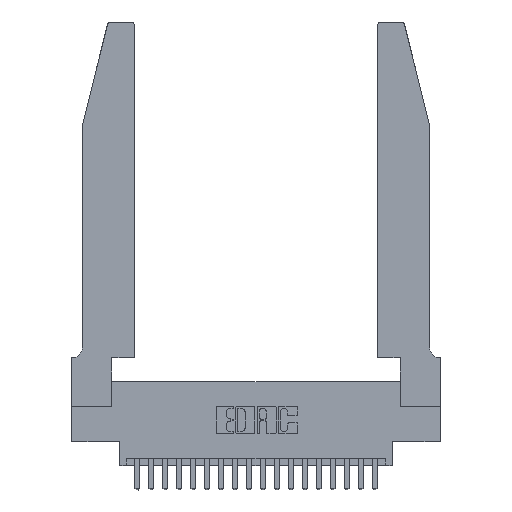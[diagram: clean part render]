
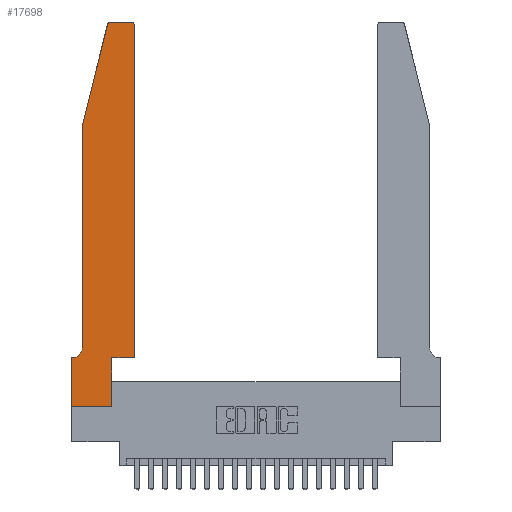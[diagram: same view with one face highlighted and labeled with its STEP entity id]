
A CAD part, top view. The second image highlights one B-rep face of the part: STEP entity #17698.
In plain terms, the highlighted planar face has unit normal (0, 0, 1).
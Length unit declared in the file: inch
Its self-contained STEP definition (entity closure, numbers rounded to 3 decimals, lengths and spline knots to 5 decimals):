
#39 = VERTEX_POINT ( 'NONE', #20597 ) ;
#129 = DIRECTION ( 'NONE',  ( 1., 0., 0. ) ) ;
#146 = LINE ( 'NONE', #2811, #18498 ) ;
#521 = EDGE_CURVE ( 'NONE', #4334, #8760, #20415, .T. ) ;
#886 = CARTESIAN_POINT ( 'NONE',  ( 0.4505, 0.35, 0.37 ) ) ;
#963 = FACE_OUTER_BOUND ( 'NONE', #15360, .T. ) ;
#997 = CARTESIAN_POINT ( 'NONE',  ( 0.0755, 2., 0.37 ) ) ;
#1043 = DIRECTION ( 'NONE',  ( -1., 0., 0. ) ) ;
#1057 = LINE ( 'NONE', #11172, #6440 ) ;
#1063 = DIRECTION ( 'NONE',  ( -1., 0., 0. ) ) ;
#1068 = VERTEX_POINT ( 'NONE', #13540 ) ;
#1978 = ORIENTED_EDGE ( 'NONE', *, *, #2964, .T. ) ;
#2248 = ORIENTED_EDGE ( 'NONE', *, *, #521, .T. ) ;
#2515 = LINE ( 'NONE', #7045, #15739 ) ;
#2811 = CARTESIAN_POINT ( 'NONE',  ( 0.0755, 0.35, 0.37 ) ) ;
#2919 = CIRCLE ( 'NONE', #5789, 0.07 ) ;
#2964 = EDGE_CURVE ( 'NONE', #6423, #7801, #2919, .T. ) ;
#3041 = DIRECTION ( 'NONE',  ( 0., 1., 0. ) ) ;
#3249 = ORIENTED_EDGE ( 'NONE', *, *, #6987, .T. ) ;
#3311 = LINE ( 'NONE', #997, #21157 ) ;
#4334 = VERTEX_POINT ( 'NONE', #6248 ) ;
#4437 = CARTESIAN_POINT ( 'NONE',  ( 0.4205, 2.75, 0.37 ) ) ;
#4625 = CARTESIAN_POINT ( 'NONE',  ( 0., 0.35, 0.37 ) ) ;
#4846 = VERTEX_POINT ( 'NONE', #6883 ) ;
#5256 = AXIS2_PLACEMENT_3D ( 'NONE', #4625, #16983, #6593 ) ;
#5789 = AXIS2_PLACEMENT_3D ( 'NONE', #18324, #9510, #1063 ) ;
#6032 = CIRCLE ( 'NONE', #10342, 0.03 ) ;
#6248 = CARTESIAN_POINT ( 'NONE',  ( 0.2865, 0., 0.37 ) ) ;
#6250 = EDGE_CURVE ( 'NONE', #8760, #12734, #2515, .T. ) ;
#6423 = VERTEX_POINT ( 'NONE', #20070 ) ;
#6440 = VECTOR ( 'NONE', #12115, 39.37008 ) ;
#6550 = EDGE_CURVE ( 'NONE', #12339, #10295, #15762, .T. ) ;
#6593 = DIRECTION ( 'NONE',  ( 1., 0., 0. ) ) ;
#6603 = VECTOR ( 'NONE', #19435, 39.37008 ) ;
#6852 = ORIENTED_EDGE ( 'NONE', *, *, #17576, .T. ) ;
#6883 = CARTESIAN_POINT ( 'NONE',  ( 0.284, 2.75, 0.37 ) ) ;
#6898 = CARTESIAN_POINT ( 'NONE',  ( 0.4205, 2.72, 0.37 ) ) ;
#6928 = EDGE_CURVE ( 'NONE', #21366, #16320, #6032, .T. ) ;
#6987 = EDGE_CURVE ( 'NONE', #39, #1068, #20617, .T. ) ;
#7045 = CARTESIAN_POINT ( 'NONE',  ( 0.4505, 0.35, 0.37 ) ) ;
#7542 = EDGE_CURVE ( 'NONE', #1068, #4334, #12728, .T. ) ;
#7801 = VERTEX_POINT ( 'NONE', #19769 ) ;
#7810 = DIRECTION ( 'NONE',  ( -1., 0., 0. ) ) ;
#7979 = ORIENTED_EDGE ( 'NONE', *, *, #18011, .T. ) ;
#8167 = CIRCLE ( 'NONE', #14293, 0.03 ) ;
#8760 = VERTEX_POINT ( 'NONE', #13416 ) ;
#8871 = DIRECTION ( 'NONE',  ( 1., 0., 0. ) ) ;
#9034 = CARTESIAN_POINT ( 'NONE',  ( 0.4505, 2.72, 0.37 ) ) ;
#9256 = CARTESIAN_POINT ( 'NONE',  ( 0.0755, 2., 0.37 ) ) ;
#9510 = DIRECTION ( 'NONE',  ( 0., 0., -1. ) ) ;
#9572 = LINE ( 'NONE', #13092, #20100 ) ;
#9945 = ORIENTED_EDGE ( 'NONE', *, *, #6550, .T. ) ;
#10111 = ORIENTED_EDGE ( 'NONE', *, *, #15379, .T. ) ;
#10263 = CARTESIAN_POINT ( 'NONE',  ( 0.25487, 2.72718, 0.37 ) ) ;
#10295 = VERTEX_POINT ( 'NONE', #19244 ) ;
#10308 = CARTESIAN_POINT ( 'NONE',  ( 0.2865, 0.35, 0.37 ) ) ;
#10338 = VECTOR ( 'NONE', #12383, 39.37008 ) ;
#10342 = AXIS2_PLACEMENT_3D ( 'NONE', #6898, #19477, #10809 ) ;
#10467 = DIRECTION ( 'NONE',  ( 0., 0., 1. ) ) ;
#10809 = DIRECTION ( 'NONE',  ( 1., 0., 0. ) ) ;
#11100 = CARTESIAN_POINT ( 'NONE',  ( 0., 0., 0.37 ) ) ;
#11172 = CARTESIAN_POINT ( 'NONE',  ( 0.4505, 0.35, 0.37 ) ) ;
#11735 = PLANE ( 'NONE',  #5256 ) ;
#12115 = DIRECTION ( 'NONE',  ( 0., 1., 0. ) ) ;
#12268 = CARTESIAN_POINT ( 'NONE',  ( 0.284, 2.72, 0.37 ) ) ;
#12339 = VERTEX_POINT ( 'NONE', #10263 ) ;
#12383 = DIRECTION ( 'NONE',  ( 1., 0., 0. ) ) ;
#12728 = LINE ( 'NONE', #15839, #10338 ) ;
#12734 = VERTEX_POINT ( 'NONE', #886 ) ;
#13092 = CARTESIAN_POINT ( 'NONE',  ( 0.2605, 2.75, 0.37 ) ) ;
#13416 = CARTESIAN_POINT ( 'NONE',  ( 0.2865, 0.35, 0.37 ) ) ;
#13540 = CARTESIAN_POINT ( 'NONE',  ( 0., 0., 0.37 ) ) ;
#14066 = EDGE_CURVE ( 'NONE', #4846, #12339, #8167, .T. ) ;
#14293 = AXIS2_PLACEMENT_3D ( 'NONE', #12268, #10467, #129 ) ;
#14517 = ORIENTED_EDGE ( 'NONE', *, *, #6928, .T. ) ;
#14849 = ORIENTED_EDGE ( 'NONE', *, *, #7542, .T. ) ;
#15151 = ORIENTED_EDGE ( 'NONE', *, *, #19884, .T. ) ;
#15360 = EDGE_LOOP ( 'NONE', ( #7979, #15621, #9945, #15151, #1978, #6852, #3249, #14849, #2248, #18235, #10111, #14517 ) ) ;
#15379 = EDGE_CURVE ( 'NONE', #12734, #21366, #1057, .T. ) ;
#15621 = ORIENTED_EDGE ( 'NONE', *, *, #14066, .T. ) ;
#15739 = VECTOR ( 'NONE', #8871, 39.37008 ) ;
#15762 = LINE ( 'NONE', #9256, #6603 ) ;
#15806 = VECTOR ( 'NONE', #3041, 39.37008 ) ;
#15839 = CARTESIAN_POINT ( 'NONE',  ( 0., 0., 0.37 ) ) ;
#16279 = DIRECTION ( 'NONE',  ( 0., -1., 0. ) ) ;
#16320 = VERTEX_POINT ( 'NONE', #4437 ) ;
#16983 = DIRECTION ( 'NONE',  ( 0., 0., 1. ) ) ;
#17576 = EDGE_CURVE ( 'NONE', #7801, #39, #146, .T. ) ;
#17698 = ADVANCED_FACE ( 'NONE', ( #963 ), #11735, .T. ) ;
#17915 = VECTOR ( 'NONE', #21372, 39.37008 ) ;
#18011 = EDGE_CURVE ( 'NONE', #16320, #4846, #9572, .T. ) ;
#18235 = ORIENTED_EDGE ( 'NONE', *, *, #6250, .T. ) ;
#18324 = CARTESIAN_POINT ( 'NONE',  ( 0.0055, 0.42, 0.37 ) ) ;
#18498 = VECTOR ( 'NONE', #7810, 39.37008 ) ;
#19244 = CARTESIAN_POINT ( 'NONE',  ( 0.0755, 2., 0.37 ) ) ;
#19435 = DIRECTION ( 'NONE',  ( -0.239, -0.971, 0. ) ) ;
#19477 = DIRECTION ( 'NONE',  ( 0., 0., 1. ) ) ;
#19769 = CARTESIAN_POINT ( 'NONE',  ( 0.0055, 0.35, 0.37 ) ) ;
#19884 = EDGE_CURVE ( 'NONE', #10295, #6423, #3311, .T. ) ;
#20070 = CARTESIAN_POINT ( 'NONE',  ( 0.0755, 0.42, 0.37 ) ) ;
#20100 = VECTOR ( 'NONE', #1043, 39.37008 ) ;
#20415 = LINE ( 'NONE', #10308, #15806 ) ;
#20597 = CARTESIAN_POINT ( 'NONE',  ( 0., 0.35, 0.37 ) ) ;
#20617 = LINE ( 'NONE', #11100, #17915 ) ;
#21157 = VECTOR ( 'NONE', #16279, 39.37008 ) ;
#21366 = VERTEX_POINT ( 'NONE', #9034 ) ;
#21372 = DIRECTION ( 'NONE',  ( 0., -1., 0. ) ) ;
